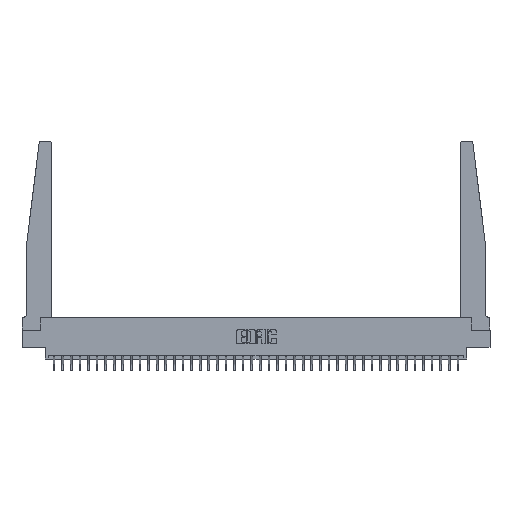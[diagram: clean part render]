
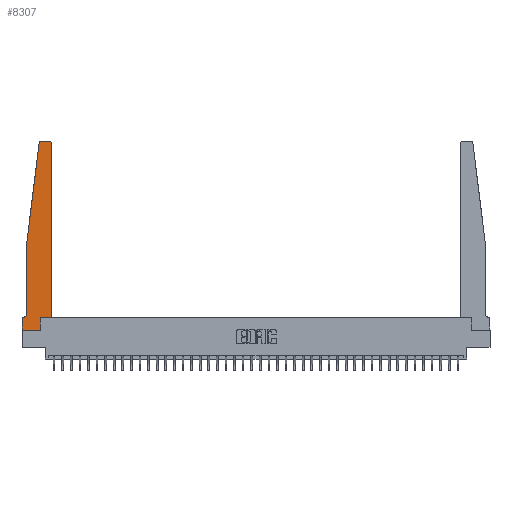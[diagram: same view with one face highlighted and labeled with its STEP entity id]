
A CAD part, top view. The second image highlights one B-rep face of the part: STEP entity #8307.
In plain terms, the highlighted planar face has unit normal (0, 0, 1).
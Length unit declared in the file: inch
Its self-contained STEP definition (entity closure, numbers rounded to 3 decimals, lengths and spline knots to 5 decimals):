
#269 = VERTEX_POINT ( 'NONE', #26690 ) ;
#1148 = LINE ( 'NONE', #19918, #27875 ) ;
#1532 = ORIENTED_EDGE ( 'NONE', *, *, #22630, .T. ) ;
#1647 = DIRECTION ( 'NONE',  ( 0., -1., 0. ) ) ;
#1817 = VERTEX_POINT ( 'NONE', #27772 ) ;
#2205 = EDGE_CURVE ( 'NONE', #2613, #25998, #24650, .T. ) ;
#2295 = DIRECTION ( 'NONE',  ( -1., 0., 0. ) ) ;
#2425 = VERTEX_POINT ( 'NONE', #22426 ) ;
#2613 = VERTEX_POINT ( 'NONE', #17729 ) ;
#4266 = VECTOR ( 'NONE', #27942, 39.37008 ) ;
#4317 = CARTESIAN_POINT ( 'NONE',  ( 0.395, 2.72, 0.37 ) ) ;
#5832 = EDGE_CURVE ( 'NONE', #25998, #9300, #8873, .T. ) ;
#6218 = DIRECTION ( 'NONE',  ( 1., 0., 0. ) ) ;
#6574 = FACE_OUTER_BOUND ( 'NONE', #11791, .T. ) ;
#6878 = EDGE_CURVE ( 'NONE', #25449, #2613, #22166, .T. ) ;
#6988 = CARTESIAN_POINT ( 'NONE',  ( 0., 0., 0.37 ) ) ;
#7115 = DIRECTION ( 'NONE',  ( 1., 0., 0. ) ) ;
#7151 = DIRECTION ( 'NONE',  ( 1., 0., 0. ) ) ;
#7172 = EDGE_CURVE ( 'NONE', #269, #24319, #22567, .T. ) ;
#7460 = VECTOR ( 'NONE', #22281, 39.37008 ) ;
#7879 = LINE ( 'NONE', #26004, #14349 ) ;
#8216 = CARTESIAN_POINT ( 'NONE',  ( 0.2605, 0., 0.37 ) ) ;
#8307 = ADVANCED_FACE ( 'NONE', ( #6574 ), #14940, .T. ) ;
#8873 = LINE ( 'NONE', #18136, #10616 ) ;
#8905 = ORIENTED_EDGE ( 'NONE', *, *, #13479, .T. ) ;
#9300 = VERTEX_POINT ( 'NONE', #13708 ) ;
#9571 = DIRECTION ( 'NONE',  ( 0., 1., 0. ) ) ;
#10616 = VECTOR ( 'NONE', #1647, 39.37008 ) ;
#10646 = ORIENTED_EDGE ( 'NONE', *, *, #19198, .T. ) ;
#10757 = AXIS2_PLACEMENT_3D ( 'NONE', #14015, #15517, #21082 ) ;
#10982 = DIRECTION ( 'NONE',  ( -1., 0., 0. ) ) ;
#11179 = VERTEX_POINT ( 'NONE', #23254 ) ;
#11383 = CARTESIAN_POINT ( 'NONE',  ( 0., 0., 0.37 ) ) ;
#11513 = CARTESIAN_POINT ( 'NONE',  ( 0.27653, 2.72, 0.37 ) ) ;
#11791 = EDGE_LOOP ( 'NONE', ( #23113, #19613, #33427, #17904, #10646, #23496, #8905, #1532, #35562, #20941, #11934, #33016 ) ) ;
#11934 = ORIENTED_EDGE ( 'NONE', *, *, #24217, .T. ) ;
#12760 = AXIS2_PLACEMENT_3D ( 'NONE', #11513, #30735, #14283 ) ;
#13479 = EDGE_CURVE ( 'NONE', #2425, #11179, #29410, .T. ) ;
#13708 = CARTESIAN_POINT ( 'NONE',  ( 0.065, 0.2375, 0.37 ) ) ;
#13740 = EDGE_CURVE ( 'NONE', #27783, #1817, #7879, .T. ) ;
#14015 = CARTESIAN_POINT ( 'NONE',  ( 0.015, 0.2375, 0.37 ) ) ;
#14283 = DIRECTION ( 'NONE',  ( 1., 0., 0. ) ) ;
#14349 = VECTOR ( 'NONE', #9571, 39.37008 ) ;
#14940 = PLANE ( 'NONE',  #21041 ) ;
#15517 = DIRECTION ( 'NONE',  ( 0., 0., -1. ) ) ;
#15858 = LINE ( 'NONE', #27105, #23146 ) ;
#16504 = CARTESIAN_POINT ( 'NONE',  ( 0.425, 0.18, 0.37 ) ) ;
#16593 = CARTESIAN_POINT ( 'NONE',  ( 0.015, 0.1875, 0.37 ) ) ;
#17184 = EDGE_CURVE ( 'NONE', #24319, #25449, #15858, .T. ) ;
#17288 = VERTEX_POINT ( 'NONE', #16504 ) ;
#17339 = VECTOR ( 'NONE', #18215, 39.37008 ) ;
#17497 = CIRCLE ( 'NONE', #10757, 0.05 ) ;
#17681 = DIRECTION ( 'NONE',  ( 1., 0., 0. ) ) ;
#17729 = CARTESIAN_POINT ( 'NONE',  ( 0.24675, 2.72367, 0.37 ) ) ;
#17824 = VECTOR ( 'NONE', #10982, 39.37008 ) ;
#17904 = ORIENTED_EDGE ( 'NONE', *, *, #5832, .T. ) ;
#18136 = CARTESIAN_POINT ( 'NONE',  ( 0.065, 1.25, 0.37 ) ) ;
#18215 = DIRECTION ( 'NONE',  ( -0.122, -0.992, 0. ) ) ;
#19198 = EDGE_CURVE ( 'NONE', #9300, #24763, #17497, .T. ) ;
#19613 = ORIENTED_EDGE ( 'NONE', *, *, #6878, .T. ) ;
#19918 = CARTESIAN_POINT ( 'NONE',  ( 0.425, 0.18, 0.37 ) ) ;
#20219 = CARTESIAN_POINT ( 'NONE',  ( 0.395, 2.75, 0.37 ) ) ;
#20941 = ORIENTED_EDGE ( 'NONE', *, *, #34686, .T. ) ;
#20998 = CARTESIAN_POINT ( 'NONE',  ( 0.065, 1.25, 0.37 ) ) ;
#21041 = AXIS2_PLACEMENT_3D ( 'NONE', #28652, #34200, #17681 ) ;
#21082 = DIRECTION ( 'NONE',  ( -1., 0., 0. ) ) ;
#22166 = CIRCLE ( 'NONE', #12760, 0.03 ) ;
#22281 = DIRECTION ( 'NONE',  ( 0., -1., 0. ) ) ;
#22426 = CARTESIAN_POINT ( 'NONE',  ( 0., 0.1875, 0.37 ) ) ;
#22567 = CIRCLE ( 'NONE', #34881, 0.03 ) ;
#22630 = EDGE_CURVE ( 'NONE', #11179, #27783, #24209, .T. ) ;
#22986 = CARTESIAN_POINT ( 'NONE',  ( 0.27653, 2.75, 0.37 ) ) ;
#23113 = ORIENTED_EDGE ( 'NONE', *, *, #17184, .T. ) ;
#23146 = VECTOR ( 'NONE', #2295, 39.37008 ) ;
#23254 = CARTESIAN_POINT ( 'NONE',  ( 0., 0., 0.37 ) ) ;
#23496 = ORIENTED_EDGE ( 'NONE', *, *, #30288, .T. ) ;
#23606 = DIRECTION ( 'NONE',  ( 0., 0., 1. ) ) ;
#24209 = LINE ( 'NONE', #6988, #25940 ) ;
#24217 = EDGE_CURVE ( 'NONE', #17288, #269, #32740, .T. ) ;
#24319 = VERTEX_POINT ( 'NONE', #20219 ) ;
#24650 = LINE ( 'NONE', #20998, #17339 ) ;
#24763 = VERTEX_POINT ( 'NONE', #16593 ) ;
#25127 = LINE ( 'NONE', #35135, #17824 ) ;
#25449 = VERTEX_POINT ( 'NONE', #22986 ) ;
#25940 = VECTOR ( 'NONE', #7115, 39.37008 ) ;
#25998 = VERTEX_POINT ( 'NONE', #33936 ) ;
#26004 = CARTESIAN_POINT ( 'NONE',  ( 0.2605, 0.18, 0.37 ) ) ;
#26690 = CARTESIAN_POINT ( 'NONE',  ( 0.425, 2.72, 0.37 ) ) ;
#27105 = CARTESIAN_POINT ( 'NONE',  ( 0.25, 2.75, 0.37 ) ) ;
#27772 = CARTESIAN_POINT ( 'NONE',  ( 0.2605, 0.18, 0.37 ) ) ;
#27783 = VERTEX_POINT ( 'NONE', #8216 ) ;
#27875 = VECTOR ( 'NONE', #6218, 39.37008 ) ;
#27942 = DIRECTION ( 'NONE',  ( 0., 1., 0. ) ) ;
#28652 = CARTESIAN_POINT ( 'NONE',  ( 0., 0.1875, 0.37 ) ) ;
#29410 = LINE ( 'NONE', #11383, #7460 ) ;
#30288 = EDGE_CURVE ( 'NONE', #24763, #2425, #25127, .T. ) ;
#30735 = DIRECTION ( 'NONE',  ( 0., 0., 1. ) ) ;
#32740 = LINE ( 'NONE', #33608, #4266 ) ;
#33016 = ORIENTED_EDGE ( 'NONE', *, *, #7172, .T. ) ;
#33427 = ORIENTED_EDGE ( 'NONE', *, *, #2205, .T. ) ;
#33608 = CARTESIAN_POINT ( 'NONE',  ( 0.425, 0.18, 0.37 ) ) ;
#33936 = CARTESIAN_POINT ( 'NONE',  ( 0.065, 1.25, 0.37 ) ) ;
#34200 = DIRECTION ( 'NONE',  ( 0., 0., 1. ) ) ;
#34686 = EDGE_CURVE ( 'NONE', #1817, #17288, #1148, .T. ) ;
#34881 = AXIS2_PLACEMENT_3D ( 'NONE', #4317, #23606, #7151 ) ;
#35135 = CARTESIAN_POINT ( 'NONE',  ( 0.065, 0.1875, 0.37 ) ) ;
#35562 = ORIENTED_EDGE ( 'NONE', *, *, #13740, .T. ) ;
